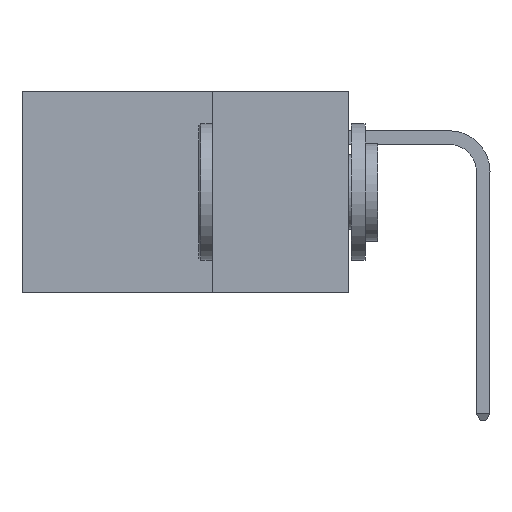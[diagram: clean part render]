
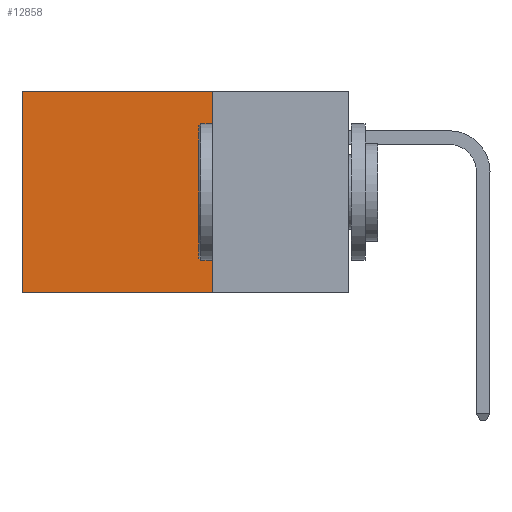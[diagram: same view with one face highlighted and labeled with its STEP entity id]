
A CAD part, left-side view. The second image highlights one B-rep face of the part: STEP entity #12858.
In plain terms, the highlighted planar face has unit normal (-1, 0, 0).
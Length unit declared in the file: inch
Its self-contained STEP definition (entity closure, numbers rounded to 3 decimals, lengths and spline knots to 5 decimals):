
#1959 = CARTESIAN_POINT ( 'NONE',  ( 0.2875, 0.25, 0. ) ) ;
#3363 = EDGE_CURVE ( 'NONE', #5394, #32306, #19760, .T. ) ;
#4633 = CARTESIAN_POINT ( 'NONE',  ( 0.2875, 0.25, -0.37 ) ) ;
#5306 = ORIENTED_EDGE ( 'NONE', *, *, #9771, .F. ) ;
#5394 = VERTEX_POINT ( 'NONE', #1959 ) ;
#5410 = CARTESIAN_POINT ( 'NONE',  ( 0.2875, 0.6, 0. ) ) ;
#8048 = VECTOR ( 'NONE', #28682, 39.37008 ) ;
#9392 = ORIENTED_EDGE ( 'NONE', *, *, #21962, .T. ) ;
#9418 = VECTOR ( 'NONE', #26899, 39.37008 ) ;
#9771 = EDGE_CURVE ( 'NONE', #13443, #12285, #31657, .T. ) ;
#11395 = CARTESIAN_POINT ( 'NONE',  ( 0.2875, 0.6, 0. ) ) ;
#12285 = VERTEX_POINT ( 'NONE', #26207 ) ;
#12858 = ADVANCED_FACE ( 'NONE', ( #29829 ), #30880, .F. ) ;
#13210 = ORIENTED_EDGE ( 'NONE', *, *, #3363, .T. ) ;
#13443 = VERTEX_POINT ( 'NONE', #18724 ) ;
#15997 = EDGE_LOOP ( 'NONE', ( #9392, #5306, #26238, #13210 ) ) ;
#16511 = DIRECTION ( 'NONE',  ( 0., 0., -1. ) ) ;
#16636 = LINE ( 'NONE', #11395, #29092 ) ;
#17855 = AXIS2_PLACEMENT_3D ( 'NONE', #18466, #18681, #20644 ) ;
#18466 = CARTESIAN_POINT ( 'NONE',  ( 0.2875, 0.25, 0. ) ) ;
#18681 = DIRECTION ( 'NONE',  ( 1., 0., 0. ) ) ;
#18724 = CARTESIAN_POINT ( 'NONE',  ( 0.2875, 0.25, -0.37 ) ) ;
#19760 = LINE ( 'NONE', #31395, #8048 ) ;
#20644 = DIRECTION ( 'NONE',  ( 0., 0., -1. ) ) ;
#20848 = EDGE_CURVE ( 'NONE', #5394, #13443, #29326, .T. ) ;
#21804 = CARTESIAN_POINT ( 'NONE',  ( 0.2875, 0.25, 0. ) ) ;
#21962 = EDGE_CURVE ( 'NONE', #32306, #12285, #16636, .T. ) ;
#25884 = VECTOR ( 'NONE', #28980, 39.37008 ) ;
#26207 = CARTESIAN_POINT ( 'NONE',  ( 0.2875, 0.6, -0.37 ) ) ;
#26238 = ORIENTED_EDGE ( 'NONE', *, *, #20848, .F. ) ;
#26899 = DIRECTION ( 'NONE',  ( 0., 1., 0. ) ) ;
#28682 = DIRECTION ( 'NONE',  ( 0., 1., 0. ) ) ;
#28980 = DIRECTION ( 'NONE',  ( 0., 0., -1. ) ) ;
#29092 = VECTOR ( 'NONE', #16511, 39.37008 ) ;
#29326 = LINE ( 'NONE', #21804, #25884 ) ;
#29829 = FACE_OUTER_BOUND ( 'NONE', #15997, .T. ) ;
#30880 = PLANE ( 'NONE',  #17855 ) ;
#31395 = CARTESIAN_POINT ( 'NONE',  ( 0.2875, 0.25, 0. ) ) ;
#31657 = LINE ( 'NONE', #4633, #9418 ) ;
#32306 = VERTEX_POINT ( 'NONE', #5410 ) ;
